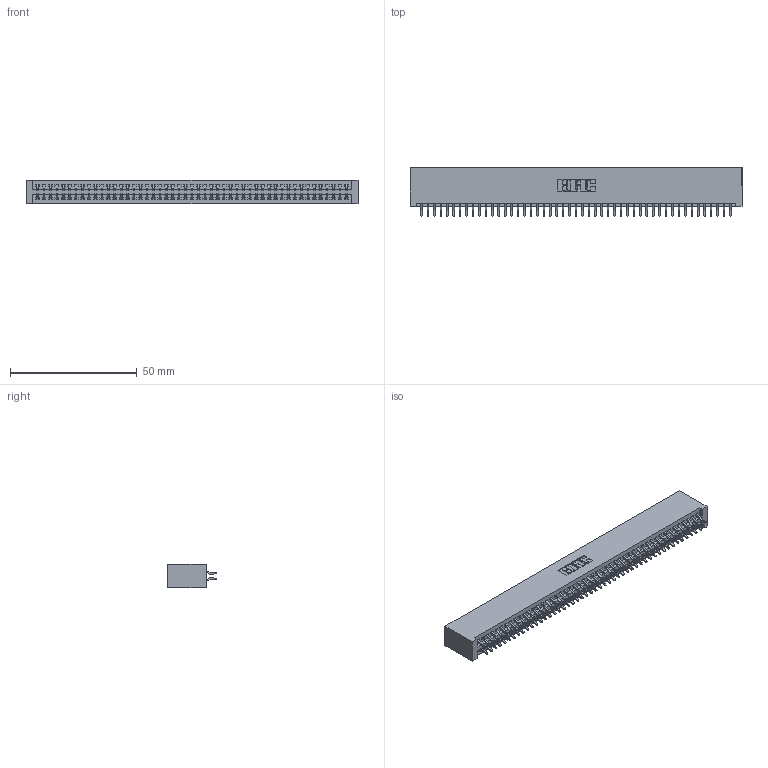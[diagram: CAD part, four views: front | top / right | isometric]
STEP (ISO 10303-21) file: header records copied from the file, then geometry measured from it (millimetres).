
FILE_DESCRIPTION (( 'STEP AP203' ), '1' );
FILE_NAME ('395-098-556-201.STEP', '2018-11-29T21:53:23', ( '' ), ( '' ), 'SwSTEP 2.0', 'SolidWorks 2016', '' );
FILE_SCHEMA (( 'CONFIG_CONTROL_DESIGN' ));
Length unit declared in the file: inch
Products named in the file (3): 345-292-001_556 Tail; 345 Part_No Mounting Lugs; 395-098-556-201
Assembly tree (99 placements, depth 2):
  395-098-556-201
    345 Part_No Mounting Lugs
    345-292-001_556 Tail  x98
Bounding box: 131.06 x 19.24 x 9.4 mm (x, y, z)
Volume: 13408.7 mm3; surface area: 20173.4 mm2
Topology: 99 solids, 99 shells, 5606 faces, 16683 edges, 10990 vertices
Faces by surface type: plane 3702, cylinder 1904
Entity records: 37447 total; most frequent: CARTESIAN_POINT 6284, ORIENTED_EDGE 6206, DIRECTION 5515, EDGE_CURVE 3103, VECTOR 2775, LINE 2775, VERTEX_POINT 2066, AXIS2_PLACEMENT_3D 1370
